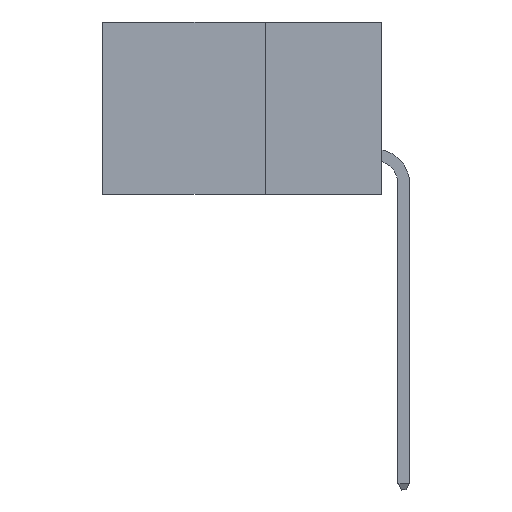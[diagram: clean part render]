
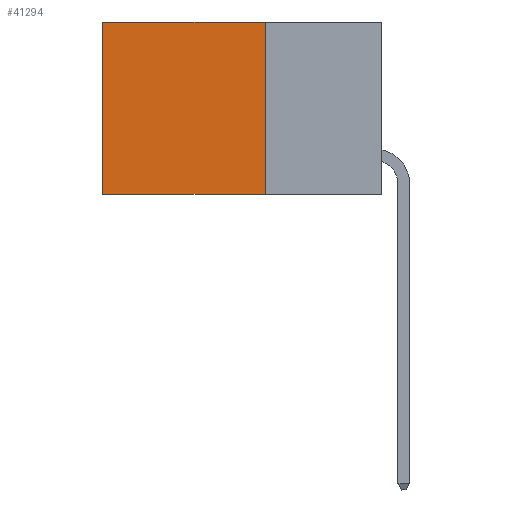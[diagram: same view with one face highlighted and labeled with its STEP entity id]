
A CAD part, left-side view. The second image highlights one B-rep face of the part: STEP entity #41294.
In plain terms, the highlighted planar face has unit normal (-1, 0, 0).
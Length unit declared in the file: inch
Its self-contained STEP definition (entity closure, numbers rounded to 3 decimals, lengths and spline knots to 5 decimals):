
#598 = LINE ( 'NONE', #3185, #24626 ) ;
#3185 = CARTESIAN_POINT ( 'NONE',  ( 0.2875, 0.25, -0.37 ) ) ;
#3596 = VECTOR ( 'NONE', #38457, 39.37008 ) ;
#3939 = VECTOR ( 'NONE', #15190, 39.37008 ) ;
#5587 = CARTESIAN_POINT ( 'NONE',  ( 0.2875, 0.25, 0. ) ) ;
#5774 = CARTESIAN_POINT ( 'NONE',  ( 0.2875, 0.6, -0.37 ) ) ;
#7149 = VERTEX_POINT ( 'NONE', #5774 ) ;
#10956 = LINE ( 'NONE', #16711, #3939 ) ;
#11195 = DIRECTION ( 'NONE',  ( 0., 0., -1. ) ) ;
#12630 = CARTESIAN_POINT ( 'NONE',  ( 0.2875, 0.25, -0.37 ) ) ;
#13834 = VERTEX_POINT ( 'NONE', #12630 ) ;
#14356 = VERTEX_POINT ( 'NONE', #43648 ) ;
#14942 = EDGE_LOOP ( 'NONE', ( #22513, #19048, #18167, #16226 ) ) ;
#15190 = DIRECTION ( 'NONE',  ( 0., 0., -1. ) ) ;
#16226 = ORIENTED_EDGE ( 'NONE', *, *, #40757, .T. ) ;
#16711 = CARTESIAN_POINT ( 'NONE',  ( 0.2875, 0.25, 0. ) ) ;
#17279 = VERTEX_POINT ( 'NONE', #5587 ) ;
#17283 = VECTOR ( 'NONE', #36589, 39.37008 ) ;
#18167 = ORIENTED_EDGE ( 'NONE', *, *, #19439, .F. ) ;
#18840 = DIRECTION ( 'NONE',  ( 1., 0., 0. ) ) ;
#19048 = ORIENTED_EDGE ( 'NONE', *, *, #30799, .F. ) ;
#19439 = EDGE_CURVE ( 'NONE', #17279, #13834, #10956, .T. ) ;
#22513 = ORIENTED_EDGE ( 'NONE', *, *, #43392, .T. ) ;
#23358 = LINE ( 'NONE', #30507, #3596 ) ;
#24626 = VECTOR ( 'NONE', #29297, 39.37008 ) ;
#29297 = DIRECTION ( 'NONE',  ( 0., 1., 0. ) ) ;
#30423 = CARTESIAN_POINT ( 'NONE',  ( 0.2875, 0.25, 0. ) ) ;
#30507 = CARTESIAN_POINT ( 'NONE',  ( 0.2875, 0.6, 0. ) ) ;
#30799 = EDGE_CURVE ( 'NONE', #13834, #7149, #598, .T. ) ;
#33537 = AXIS2_PLACEMENT_3D ( 'NONE', #30423, #18840, #11195 ) ;
#36589 = DIRECTION ( 'NONE',  ( 0., 1., 0. ) ) ;
#38457 = DIRECTION ( 'NONE',  ( 0., 0., -1. ) ) ;
#40102 = FACE_OUTER_BOUND ( 'NONE', #14942, .T. ) ;
#40635 = CARTESIAN_POINT ( 'NONE',  ( 0.2875, 0.25, 0. ) ) ;
#40757 = EDGE_CURVE ( 'NONE', #17279, #14356, #47170, .T. ) ;
#41056 = PLANE ( 'NONE',  #33537 ) ;
#41294 = ADVANCED_FACE ( 'NONE', ( #40102 ), #41056, .F. ) ;
#43392 = EDGE_CURVE ( 'NONE', #14356, #7149, #23358, .T. ) ;
#43648 = CARTESIAN_POINT ( 'NONE',  ( 0.2875, 0.6, 0. ) ) ;
#47170 = LINE ( 'NONE', #40635, #17283 ) ;
